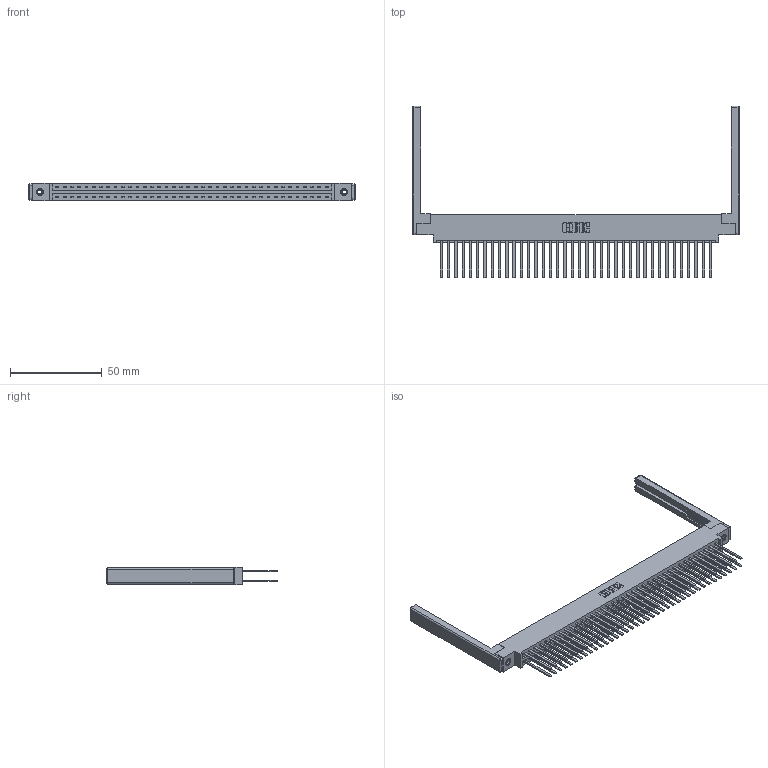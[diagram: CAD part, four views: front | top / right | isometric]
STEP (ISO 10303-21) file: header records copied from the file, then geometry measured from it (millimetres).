
FILE_DESCRIPTION (( 'STEP AP203' ), '1' );
FILE_NAME ('387-076-544-868.STEP', '2019-10-22T04:10:50', ( '' ), ( '' ), 'SwSTEP 2.0', 'SolidWorks 2016', '' );
FILE_SCHEMA (( 'CONFIG_CONTROL_DESIGN' ));
Length unit declared in the file: inch
Products named in the file (5): 307-220-068; 345-292-001_345-293-144; 337 Part_0.170 Offset - 0.156 Dia-TI; 387-076-544-868; 345-250-001_345-250-001-102
Assembly tree (81 placements, depth 2):
  387-076-544-868
    337 Part_0.170 Offset - 0.156 Dia-TI
    345-292-001_345-293-144  x76
    345-250-001_345-250-001-102  x2
    307-220-068  x2
Bounding box: 178 x 93.35 x 9.4 mm (x, y, z)
Volume: 24038.8 mm3; surface area: 29802.6 mm2
Topology: 81 solids, 81 shells, 3920 faces, 11581 edges, 7598 vertices
Faces by surface type: plane 2746, cylinder 1150, cone 12, sphere 8, torus 4
Entity records: 32688 total; most frequent: CARTESIAN_POINT 5475, ORIENTED_EDGE 5400, DIRECTION 4730, EDGE_CURVE 2700, LINE 2526, VECTOR 2526, VERTEX_POINT 1790, AXIS2_PLACEMENT_3D 1102
